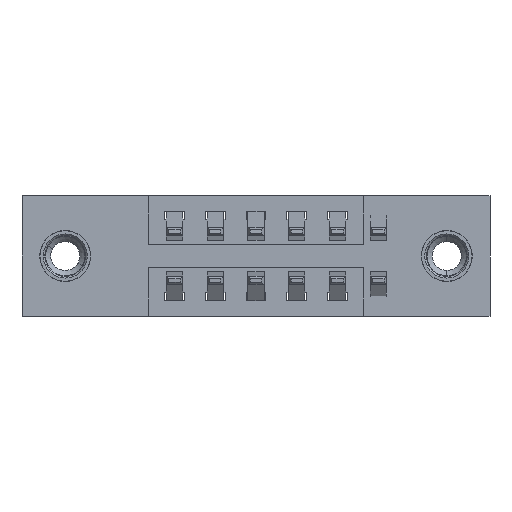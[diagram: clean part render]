
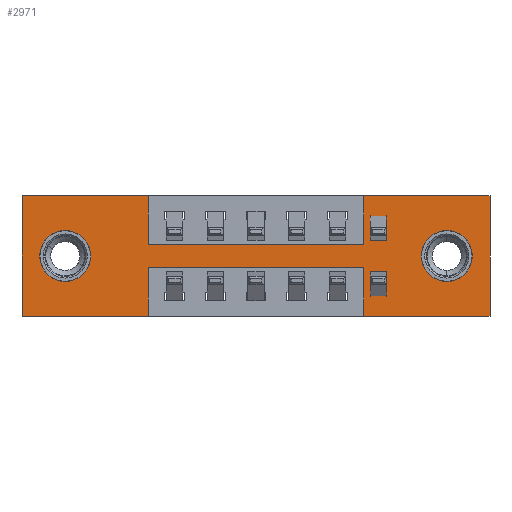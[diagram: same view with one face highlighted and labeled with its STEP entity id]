
A CAD part, front view. The second image highlights one B-rep face of the part: STEP entity #2971.
In plain terms, the highlighted planar face has unit normal (0, -1, 0).
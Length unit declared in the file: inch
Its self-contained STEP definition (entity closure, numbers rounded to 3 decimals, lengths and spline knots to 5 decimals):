
#57 = VECTOR ( 'NONE', #4831, 39.37008 ) ;
#147 = CARTESIAN_POINT ( 'NONE',  ( 0., 0., 0. ) ) ;
#150 = VERTEX_POINT ( 'NONE', #1764 ) ;
#268 = VERTEX_POINT ( 'NONE', #4828 ) ;
#289 = CIRCLE ( 'NONE', #4467, 0.078 ) ;
#291 = EDGE_CURVE ( 'NONE', #6432, #9382, #8587, .T. ) ;
#556 = ORIENTED_EDGE ( 'NONE', *, *, #6600, .T. ) ;
#684 = CARTESIAN_POINT ( 'NONE',  ( 1.435, 0., 0. ) ) ;
#764 = EDGE_LOOP ( 'NONE', ( #5578, #3866, #2279, #8346, #2204, #5444, #6183, #9096, #8615, #9226, #7227, #4587 ) ) ;
#831 = DIRECTION ( 'NONE',  ( 0., 0., 1. ) ) ;
#932 = DIRECTION ( 'NONE',  ( 0., 1., 0. ) ) ;
#1060 = AXIS2_PLACEMENT_3D ( 'NONE', #5365, #1682, #7580 ) ;
#1144 = LINE ( 'NONE', #7713, #57 ) ;
#1150 = VERTEX_POINT ( 'NONE', #4098 ) ;
#1190 = DIRECTION ( 'NONE',  ( 1., 0., 0. ) ) ;
#1247 = LINE ( 'NONE', #3305, #8939 ) ;
#1488 = DIRECTION ( 'NONE',  ( 0., 1., 0. ) ) ;
#1557 = DIRECTION ( 'NONE',  ( -1., 0., 0. ) ) ;
#1682 = DIRECTION ( 'NONE',  ( 0., 1., 0. ) ) ;
#1730 = CARTESIAN_POINT ( 'NONE',  ( 0., 0., -0.37 ) ) ;
#1744 = DIRECTION ( 'NONE',  ( 0., 0., -1. ) ) ;
#1762 = EDGE_CURVE ( 'NONE', #2710, #7907, #8228, .T. ) ;
#1764 = CARTESIAN_POINT ( 'NONE',  ( 1.0475, 0., 0. ) ) ;
#1829 = CARTESIAN_POINT ( 'NONE',  ( 0.3875, 0., -0.37 ) ) ;
#2006 = FACE_BOUND ( 'NONE', #4740, .T. ) ;
#2030 = ORIENTED_EDGE ( 'NONE', *, *, #4580, .T. ) ;
#2204 = ORIENTED_EDGE ( 'NONE', *, *, #4036, .F. ) ;
#2279 = ORIENTED_EDGE ( 'NONE', *, *, #7560, .F. ) ;
#2325 = CARTESIAN_POINT ( 'NONE',  ( 0., 0., -0.37 ) ) ;
#2438 = CARTESIAN_POINT ( 'NONE',  ( 0.3875, 0., 0. ) ) ;
#2545 = VERTEX_POINT ( 'NONE', #4850 ) ;
#2562 = DIRECTION ( 'NONE',  ( 1., 0., 0. ) ) ;
#2583 = AXIS2_PLACEMENT_3D ( 'NONE', #9341, #2722, #9293 ) ;
#2645 = VERTEX_POINT ( 'NONE', #3605 ) ;
#2710 = VERTEX_POINT ( 'NONE', #6574 ) ;
#2719 = VECTOR ( 'NONE', #1744, 39.37008 ) ;
#2722 = DIRECTION ( 'NONE',  ( 0., -1., 0. ) ) ;
#2752 = LINE ( 'NONE', #9232, #8151 ) ;
#2805 = VERTEX_POINT ( 'NONE', #1730 ) ;
#2818 = DIRECTION ( 'NONE',  ( 0., 0., -1. ) ) ;
#2846 = VERTEX_POINT ( 'NONE', #2438 ) ;
#2887 = EDGE_CURVE ( 'NONE', #2645, #7806, #5221, .T. ) ;
#2963 = CARTESIAN_POINT ( 'NONE',  ( 0.3875, 0., -0.22 ) ) ;
#2971 = ADVANCED_FACE ( 'NONE', ( #6376, #2006, #8647 ), #4186, .T. ) ;
#3008 = EDGE_CURVE ( 'NONE', #2545, #2805, #1247, .T. ) ;
#3046 = DIRECTION ( 'NONE',  ( 0., 0., 1. ) ) ;
#3122 = EDGE_CURVE ( 'NONE', #268, #5906, #7240, .T. ) ;
#3255 = EDGE_LOOP ( 'NONE', ( #9244, #556 ) ) ;
#3305 = CARTESIAN_POINT ( 'NONE',  ( 0., 0., -0.37 ) ) ;
#3410 = CARTESIAN_POINT ( 'NONE',  ( 1.0475, 0., -0.15 ) ) ;
#3496 = VECTOR ( 'NONE', #6616, 39.37008 ) ;
#3556 = CARTESIAN_POINT ( 'NONE',  ( 1.3025, 0., -0.185 ) ) ;
#3605 = CARTESIAN_POINT ( 'NONE',  ( 1.3025, 0., -0.107 ) ) ;
#3664 = EDGE_CURVE ( 'NONE', #2846, #6432, #8318, .T. ) ;
#3708 = DIRECTION ( 'NONE',  ( 1., 0., 0. ) ) ;
#3728 = LINE ( 'NONE', #147, #5171 ) ;
#3866 = ORIENTED_EDGE ( 'NONE', *, *, #3122, .F. ) ;
#3926 = VECTOR ( 'NONE', #4918, 39.37008 ) ;
#4006 = CARTESIAN_POINT ( 'NONE',  ( 0.3875, 0., 0. ) ) ;
#4036 = EDGE_CURVE ( 'NONE', #7509, #2710, #7278, .T. ) ;
#4084 = LINE ( 'NONE', #1829, #8813 ) ;
#4098 = CARTESIAN_POINT ( 'NONE',  ( 0., 0., 0. ) ) ;
#4186 = PLANE ( 'NONE',  #2583 ) ;
#4194 = CARTESIAN_POINT ( 'NONE',  ( 1.3025, 0., -0.263 ) ) ;
#4304 = EDGE_CURVE ( 'NONE', #1150, #2846, #2752, .T. ) ;
#4447 = VECTOR ( 'NONE', #5818, 39.37008 ) ;
#4467 = AXIS2_PLACEMENT_3D ( 'NONE', #8808, #6688, #5118 ) ;
#4486 = CARTESIAN_POINT ( 'NONE',  ( 0.1325, 0., -0.107 ) ) ;
#4580 = EDGE_CURVE ( 'NONE', #9594, #9493, #9110, .T. ) ;
#4587 = ORIENTED_EDGE ( 'NONE', *, *, #3008, .F. ) ;
#4740 = EDGE_LOOP ( 'NONE', ( #7055, #2030 ) ) ;
#4828 = CARTESIAN_POINT ( 'NONE',  ( 1.0475, 0., -0.22 ) ) ;
#4831 = DIRECTION ( 'NONE',  ( 0., 0., 1. ) ) ;
#4850 = CARTESIAN_POINT ( 'NONE',  ( 0.3875, 0., -0.37 ) ) ;
#4901 = EDGE_CURVE ( 'NONE', #9493, #9594, #289, .T. ) ;
#4918 = DIRECTION ( 'NONE',  ( 0., 0., 1. ) ) ;
#5019 = VECTOR ( 'NONE', #831, 39.37008 ) ;
#5051 = LINE ( 'NONE', #7993, #3926 ) ;
#5118 = DIRECTION ( 'NONE',  ( 0., 0., 1. ) ) ;
#5171 = VECTOR ( 'NONE', #3708, 39.37008 ) ;
#5221 = CIRCLE ( 'NONE', #1060, 0.078 ) ;
#5365 = CARTESIAN_POINT ( 'NONE',  ( 1.3025, 0., -0.185 ) ) ;
#5444 = ORIENTED_EDGE ( 'NONE', *, *, #7624, .F. ) ;
#5578 = ORIENTED_EDGE ( 'NONE', *, *, #5668, .F. ) ;
#5668 = EDGE_CURVE ( 'NONE', #5906, #2545, #4084, .T. ) ;
#5679 = AXIS2_PLACEMENT_3D ( 'NONE', #8323, #932, #3046 ) ;
#5818 = DIRECTION ( 'NONE',  ( -1., 0., 0. ) ) ;
#5906 = VERTEX_POINT ( 'NONE', #9122 ) ;
#6104 = AXIS2_PLACEMENT_3D ( 'NONE', #3556, #1488, #2818 ) ;
#6183 = ORIENTED_EDGE ( 'NONE', *, *, #7374, .F. ) ;
#6283 = DIRECTION ( 'NONE',  ( 0., 0., -1. ) ) ;
#6376 = FACE_BOUND ( 'NONE', #3255, .T. ) ;
#6432 = VERTEX_POINT ( 'NONE', #7068 ) ;
#6574 = CARTESIAN_POINT ( 'NONE',  ( 1.435, 0., -0.37 ) ) ;
#6600 = EDGE_CURVE ( 'NONE', #7806, #2645, #7792, .T. ) ;
#6616 = DIRECTION ( 'NONE',  ( 0., 0., -1. ) ) ;
#6688 = DIRECTION ( 'NONE',  ( 0., 1., 0. ) ) ;
#6773 = CARTESIAN_POINT ( 'NONE',  ( 0.1325, 0., -0.263 ) ) ;
#7055 = ORIENTED_EDGE ( 'NONE', *, *, #4901, .T. ) ;
#7068 = CARTESIAN_POINT ( 'NONE',  ( 0.3875, 0., -0.15 ) ) ;
#7150 = DIRECTION ( 'NONE',  ( -1., 0., 0. ) ) ;
#7227 = ORIENTED_EDGE ( 'NONE', *, *, #7754, .F. ) ;
#7240 = LINE ( 'NONE', #2963, #4447 ) ;
#7278 = LINE ( 'NONE', #684, #3496 ) ;
#7374 = EDGE_CURVE ( 'NONE', #9382, #150, #1144, .T. ) ;
#7458 = LINE ( 'NONE', #7559, #5019 ) ;
#7509 = VERTEX_POINT ( 'NONE', #9561 ) ;
#7559 = CARTESIAN_POINT ( 'NONE',  ( 0., 0., 0. ) ) ;
#7560 = EDGE_CURVE ( 'NONE', #7907, #268, #5051, .T. ) ;
#7580 = DIRECTION ( 'NONE',  ( 0., 0., -1. ) ) ;
#7624 = EDGE_CURVE ( 'NONE', #150, #7509, #3728, .T. ) ;
#7713 = CARTESIAN_POINT ( 'NONE',  ( 1.0475, 0., 0. ) ) ;
#7754 = EDGE_CURVE ( 'NONE', #2805, #1150, #7458, .T. ) ;
#7792 = CIRCLE ( 'NONE', #6104, 0.078 ) ;
#7806 = VERTEX_POINT ( 'NONE', #4194 ) ;
#7907 = VERTEX_POINT ( 'NONE', #9538 ) ;
#7911 = VECTOR ( 'NONE', #1190, 39.37008 ) ;
#7993 = CARTESIAN_POINT ( 'NONE',  ( 1.0475, 0., -0.37 ) ) ;
#8151 = VECTOR ( 'NONE', #2562, 39.37008 ) ;
#8228 = LINE ( 'NONE', #2325, #8578 ) ;
#8318 = LINE ( 'NONE', #4006, #2719 ) ;
#8323 = CARTESIAN_POINT ( 'NONE',  ( 0.1325, 0., -0.185 ) ) ;
#8346 = ORIENTED_EDGE ( 'NONE', *, *, #1762, .F. ) ;
#8578 = VECTOR ( 'NONE', #1557, 39.37008 ) ;
#8587 = LINE ( 'NONE', #9468, #7911 ) ;
#8615 = ORIENTED_EDGE ( 'NONE', *, *, #3664, .F. ) ;
#8647 = FACE_OUTER_BOUND ( 'NONE', #764, .T. ) ;
#8808 = CARTESIAN_POINT ( 'NONE',  ( 0.1325, 0., -0.185 ) ) ;
#8813 = VECTOR ( 'NONE', #6283, 39.37008 ) ;
#8939 = VECTOR ( 'NONE', #7150, 39.37008 ) ;
#9096 = ORIENTED_EDGE ( 'NONE', *, *, #291, .F. ) ;
#9110 = CIRCLE ( 'NONE', #5679, 0.078 ) ;
#9122 = CARTESIAN_POINT ( 'NONE',  ( 0.3875, 0., -0.22 ) ) ;
#9226 = ORIENTED_EDGE ( 'NONE', *, *, #4304, .F. ) ;
#9232 = CARTESIAN_POINT ( 'NONE',  ( 0., 0., 0. ) ) ;
#9244 = ORIENTED_EDGE ( 'NONE', *, *, #2887, .T. ) ;
#9293 = DIRECTION ( 'NONE',  ( 0., 0., -1. ) ) ;
#9341 = CARTESIAN_POINT ( 'NONE',  ( 0., 0., -0.37 ) ) ;
#9382 = VERTEX_POINT ( 'NONE', #3410 ) ;
#9468 = CARTESIAN_POINT ( 'NONE',  ( 0.3875, 0., -0.15 ) ) ;
#9493 = VERTEX_POINT ( 'NONE', #4486 ) ;
#9538 = CARTESIAN_POINT ( 'NONE',  ( 1.0475, 0., -0.37 ) ) ;
#9561 = CARTESIAN_POINT ( 'NONE',  ( 1.435, 0., 0. ) ) ;
#9594 = VERTEX_POINT ( 'NONE', #6773 ) ;
